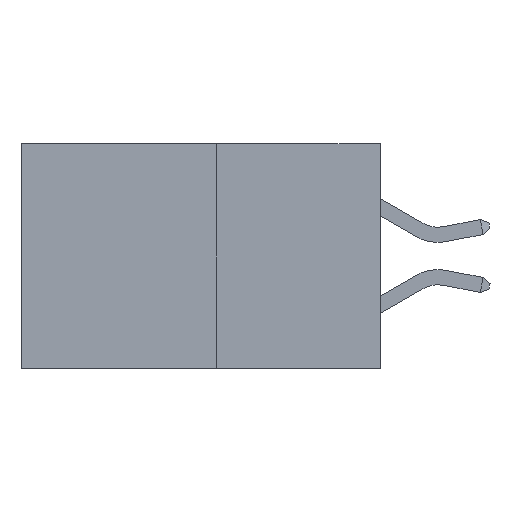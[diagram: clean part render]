
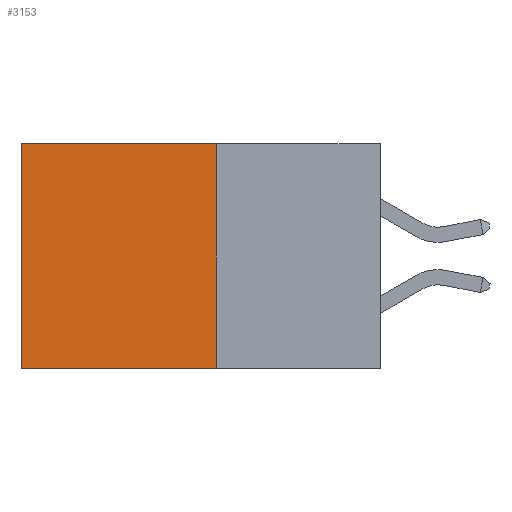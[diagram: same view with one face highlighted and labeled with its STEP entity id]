
A CAD part, left-side view. The second image highlights one B-rep face of the part: STEP entity #3153.
In plain terms, the highlighted planar face has unit normal (-1, 0, 0).
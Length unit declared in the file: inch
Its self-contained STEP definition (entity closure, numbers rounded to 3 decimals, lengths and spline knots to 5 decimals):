
#491 = CARTESIAN_POINT ( 'NONE',  ( 0.277, 0.27, -0.37 ) ) ;
#497 = ORIENTED_EDGE ( 'NONE', *, *, #11774, .F. ) ;
#1707 = VERTEX_POINT ( 'NONE', #8900 ) ;
#2794 = CARTESIAN_POINT ( 'NONE',  ( 0.277, 0.59, -0.37 ) ) ;
#2834 = CARTESIAN_POINT ( 'NONE',  ( 0.277, 0.27, -0.37 ) ) ;
#3153 = ADVANCED_FACE ( 'NONE', ( #22877 ), #6356, .F. ) ;
#4519 = CARTESIAN_POINT ( 'NONE',  ( 0.277, 0.27, -0.37 ) ) ;
#5001 = VERTEX_POINT ( 'NONE', #9124 ) ;
#5692 = LINE ( 'NONE', #491, #19609 ) ;
#6021 = VECTOR ( 'NONE', #11980, 39.37008 ) ;
#6187 = DIRECTION ( 'NONE',  ( 0., 0., -1. ) ) ;
#6356 = PLANE ( 'NONE',  #21016 ) ;
#7908 = CARTESIAN_POINT ( 'NONE',  ( 0.277, 0.27, -0.37 ) ) ;
#8201 = DIRECTION ( 'NONE',  ( 0., 0., -1. ) ) ;
#8900 = CARTESIAN_POINT ( 'NONE',  ( 0.277, 0.27, 0. ) ) ;
#9124 = CARTESIAN_POINT ( 'NONE',  ( 0.277, 0.59, 0. ) ) ;
#9233 = VECTOR ( 'NONE', #11770, 39.37008 ) ;
#9355 = VECTOR ( 'NONE', #22488, 39.37008 ) ;
#11770 = DIRECTION ( 'NONE',  ( 0., 1., 0. ) ) ;
#11774 = EDGE_CURVE ( 'NONE', #1707, #20421, #5692, .T. ) ;
#11794 = DIRECTION ( 'NONE',  ( 1., 0., 0. ) ) ;
#11980 = DIRECTION ( 'NONE',  ( 0., 1., 0. ) ) ;
#12042 = ORIENTED_EDGE ( 'NONE', *, *, #21487, .T. ) ;
#14142 = LINE ( 'NONE', #20613, #9355 ) ;
#14593 = ORIENTED_EDGE ( 'NONE', *, *, #16837, .F. ) ;
#16837 = EDGE_CURVE ( 'NONE', #20421, #19509, #19969, .T. ) ;
#19092 = EDGE_CURVE ( 'NONE', #5001, #19509, #14142, .T. ) ;
#19509 = VERTEX_POINT ( 'NONE', #2794 ) ;
#19609 = VECTOR ( 'NONE', #6187, 39.37008 ) ;
#19969 = LINE ( 'NONE', #2834, #6021 ) ;
#20421 = VERTEX_POINT ( 'NONE', #7908 ) ;
#20613 = CARTESIAN_POINT ( 'NONE',  ( 0.277, 0.59, -0.37 ) ) ;
#21016 = AXIS2_PLACEMENT_3D ( 'NONE', #4519, #11794, #8201 ) ;
#21454 = ORIENTED_EDGE ( 'NONE', *, *, #19092, .T. ) ;
#21487 = EDGE_CURVE ( 'NONE', #1707, #5001, #23145, .T. ) ;
#22488 = DIRECTION ( 'NONE',  ( 0., 0., -1. ) ) ;
#22673 = CARTESIAN_POINT ( 'NONE',  ( 0.277, 0.27, 0. ) ) ;
#22877 = FACE_OUTER_BOUND ( 'NONE', #23442, .T. ) ;
#23145 = LINE ( 'NONE', #22673, #9233 ) ;
#23442 = EDGE_LOOP ( 'NONE', ( #21454, #14593, #497, #12042 ) ) ;
